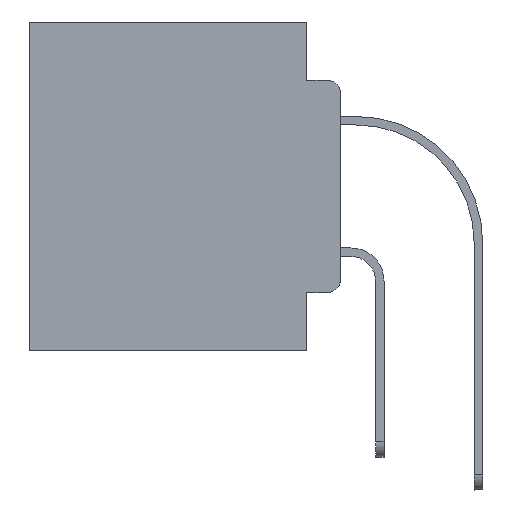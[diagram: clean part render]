
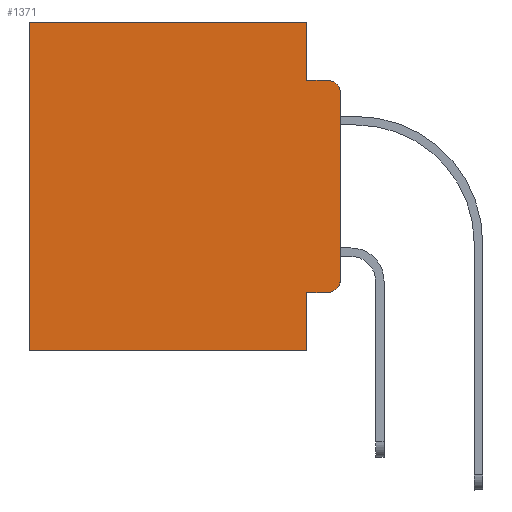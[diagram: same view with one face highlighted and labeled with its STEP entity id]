
A CAD part, left-side view. The second image highlights one B-rep face of the part: STEP entity #1371.
In plain terms, the highlighted planar face has unit normal (-1, 0, 0).
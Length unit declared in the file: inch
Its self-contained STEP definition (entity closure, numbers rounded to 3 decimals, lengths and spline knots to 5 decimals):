
#343 = CIRCLE ( 'NONE', #4957, 0.02 ) ;
#799 = ORIENTED_EDGE ( 'NONE', *, *, #14631, .F. ) ;
#1192 = VERTEX_POINT ( 'NONE', #25432 ) ;
#1208 = DIRECTION ( 'NONE',  ( -1., 0., 0. ) ) ;
#1371 = ADVANCED_FACE ( 'NONE', ( #18163 ), #7009, .F. ) ;
#1827 = CARTESIAN_POINT ( 'NONE',  ( 0.298, 0.473, 0. ) ) ;
#1996 = VECTOR ( 'NONE', #17008, 39.37008 ) ;
#2015 = CARTESIAN_POINT ( 'NONE',  ( 0.298, 0.02, -0.0885 ) ) ;
#2029 = VECTOR ( 'NONE', #18880, 39.37008 ) ;
#2090 = CARTESIAN_POINT ( 'NONE',  ( 0.298, 0.051, -0.0885 ) ) ;
#2431 = ORIENTED_EDGE ( 'NONE', *, *, #2846, .F. ) ;
#2846 = EDGE_CURVE ( 'NONE', #16606, #1192, #27427, .T. ) ;
#3005 = LINE ( 'NONE', #22962, #22489 ) ;
#3409 = LINE ( 'NONE', #25404, #16295 ) ;
#3553 = VECTOR ( 'NONE', #12949, 39.37008 ) ;
#4957 = AXIS2_PLACEMENT_3D ( 'NONE', #23036, #27958, #8124 ) ;
#5821 = CARTESIAN_POINT ( 'NONE',  ( 0.298, 0.473, -0.5 ) ) ;
#5827 = CARTESIAN_POINT ( 'NONE',  ( 0.298, 0.473, 0. ) ) ;
#5857 = CARTESIAN_POINT ( 'NONE',  ( 0.298, 0.051, 0. ) ) ;
#6197 = EDGE_CURVE ( 'NONE', #16606, #11901, #17160, .T. ) ;
#7002 = ORIENTED_EDGE ( 'NONE', *, *, #21749, .T. ) ;
#7009 = PLANE ( 'NONE',  #13203 ) ;
#7508 = AXIS2_PLACEMENT_3D ( 'NONE', #25937, #1208, #16677 ) ;
#7750 = EDGE_CURVE ( 'NONE', #13371, #10066, #3409, .T. ) ;
#8124 = DIRECTION ( 'NONE',  ( 0., 0., -1. ) ) ;
#8368 = EDGE_CURVE ( 'NONE', #13371, #9900, #26785, .T. ) ;
#9118 = ORIENTED_EDGE ( 'NONE', *, *, #15747, .F. ) ;
#9635 = ORIENTED_EDGE ( 'NONE', *, *, #8368, .T. ) ;
#9900 = VERTEX_POINT ( 'NONE', #28037 ) ;
#10066 = VERTEX_POINT ( 'NONE', #11797 ) ;
#10660 = VERTEX_POINT ( 'NONE', #2015 ) ;
#11450 = CARTESIAN_POINT ( 'NONE',  ( 0.298, 0., -0.3915 ) ) ;
#11471 = EDGE_CURVE ( 'NONE', #1192, #10660, #12794, .T. ) ;
#11503 = DIRECTION ( 'NONE',  ( 0., 0., -1. ) ) ;
#11797 = CARTESIAN_POINT ( 'NONE',  ( 0.298, 0.051, -0.5 ) ) ;
#11901 = VERTEX_POINT ( 'NONE', #5827 ) ;
#12794 = LINE ( 'NONE', #2090, #1996 ) ;
#12949 = DIRECTION ( 'NONE',  ( 0., 0., -1. ) ) ;
#13203 = AXIS2_PLACEMENT_3D ( 'NONE', #26996, #24537, #11503 ) ;
#13371 = VERTEX_POINT ( 'NONE', #17967 ) ;
#13709 = ORIENTED_EDGE ( 'NONE', *, *, #11471, .F. ) ;
#14592 = CARTESIAN_POINT ( 'NONE',  ( 0.298, 0.051, 0. ) ) ;
#14631 = EDGE_CURVE ( 'NONE', #16516, #20895, #19296, .T. ) ;
#15090 = CARTESIAN_POINT ( 'NONE',  ( 0.298, 0., 0. ) ) ;
#15747 = EDGE_CURVE ( 'NONE', #10066, #21644, #3005, .T. ) ;
#15908 = CARTESIAN_POINT ( 'NONE',  ( 0.298, 0., -0.1085 ) ) ;
#16185 = EDGE_CURVE ( 'NONE', #16516, #10660, #343, .T. ) ;
#16295 = VECTOR ( 'NONE', #22674, 39.37008 ) ;
#16396 = ORIENTED_EDGE ( 'NONE', *, *, #17263, .T. ) ;
#16516 = VERTEX_POINT ( 'NONE', #15908 ) ;
#16606 = VERTEX_POINT ( 'NONE', #14592 ) ;
#16677 = DIRECTION ( 'NONE',  ( 0., 0., -1. ) ) ;
#17008 = DIRECTION ( 'NONE',  ( 0., -1., 0. ) ) ;
#17160 = LINE ( 'NONE', #19471, #25208 ) ;
#17263 = EDGE_CURVE ( 'NONE', #11901, #21644, #19053, .T. ) ;
#17967 = CARTESIAN_POINT ( 'NONE',  ( 0.298, 0.051, -0.4115 ) ) ;
#18141 = VECTOR ( 'NONE', #20125, 39.37008 ) ;
#18163 = FACE_OUTER_BOUND ( 'NONE', #22748, .T. ) ;
#18880 = DIRECTION ( 'NONE',  ( 0., 0., -1. ) ) ;
#19053 = LINE ( 'NONE', #1827, #3553 ) ;
#19296 = LINE ( 'NONE', #15090, #21661 ) ;
#19471 = CARTESIAN_POINT ( 'NONE',  ( 0.298, 0., 0. ) ) ;
#19993 = CIRCLE ( 'NONE', #7508, 0.02 ) ;
#20125 = DIRECTION ( 'NONE',  ( 0., -1., 0. ) ) ;
#20508 = DIRECTION ( 'NONE',  ( 0., 1., 0. ) ) ;
#20613 = ORIENTED_EDGE ( 'NONE', *, *, #7750, .F. ) ;
#20895 = VERTEX_POINT ( 'NONE', #11450 ) ;
#21644 = VERTEX_POINT ( 'NONE', #5821 ) ;
#21661 = VECTOR ( 'NONE', #28126, 39.37008 ) ;
#21749 = EDGE_CURVE ( 'NONE', #9900, #20895, #19993, .T. ) ;
#22489 = VECTOR ( 'NONE', #20508, 39.37008 ) ;
#22674 = DIRECTION ( 'NONE',  ( 0., 0., -1. ) ) ;
#22748 = EDGE_LOOP ( 'NONE', ( #799, #25082, #13709, #2431, #28538, #16396, #9118, #20613, #9635, #7002 ) ) ;
#22962 = CARTESIAN_POINT ( 'NONE',  ( 0.298, 0., -0.5 ) ) ;
#23036 = CARTESIAN_POINT ( 'NONE',  ( 0.298, 0.02, -0.1085 ) ) ;
#24190 = CARTESIAN_POINT ( 'NONE',  ( 0.298, 0.051, -0.4115 ) ) ;
#24537 = DIRECTION ( 'NONE',  ( 1., 0., 0. ) ) ;
#25082 = ORIENTED_EDGE ( 'NONE', *, *, #16185, .T. ) ;
#25208 = VECTOR ( 'NONE', #28027, 39.37008 ) ;
#25404 = CARTESIAN_POINT ( 'NONE',  ( 0.298, 0.051, 0. ) ) ;
#25432 = CARTESIAN_POINT ( 'NONE',  ( 0.298, 0.051, -0.0885 ) ) ;
#25937 = CARTESIAN_POINT ( 'NONE',  ( 0.298, 0.02, -0.3915 ) ) ;
#26785 = LINE ( 'NONE', #24190, #18141 ) ;
#26996 = CARTESIAN_POINT ( 'NONE',  ( 0.298, 0., 0. ) ) ;
#27427 = LINE ( 'NONE', #5857, #2029 ) ;
#27958 = DIRECTION ( 'NONE',  ( -1., 0., 0. ) ) ;
#28027 = DIRECTION ( 'NONE',  ( 0., 1., 0. ) ) ;
#28037 = CARTESIAN_POINT ( 'NONE',  ( 0.298, 0.02, -0.4115 ) ) ;
#28126 = DIRECTION ( 'NONE',  ( 0., 0., -1. ) ) ;
#28538 = ORIENTED_EDGE ( 'NONE', *, *, #6197, .T. ) ;
